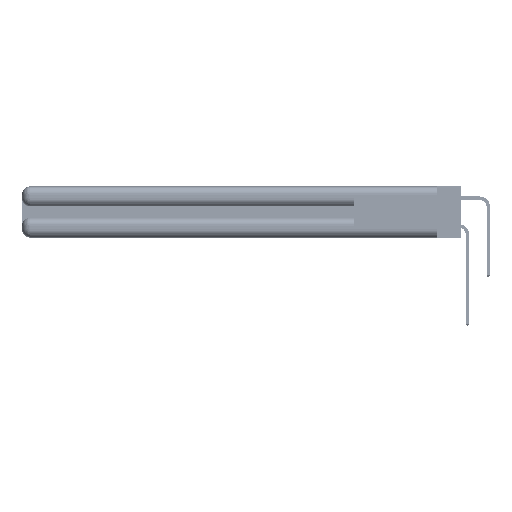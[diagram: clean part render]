
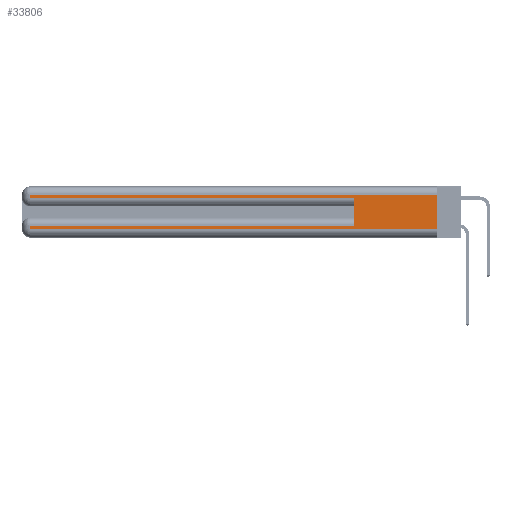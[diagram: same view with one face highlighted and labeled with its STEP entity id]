
A CAD part, left-side view. The second image highlights one B-rep face of the part: STEP entity #33806.
In plain terms, the highlighted planar face has unit normal (-1, 0, 0).
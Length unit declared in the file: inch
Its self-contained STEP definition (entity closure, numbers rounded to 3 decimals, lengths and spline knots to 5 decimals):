
#61 = CARTESIAN_POINT ( 'NONE',  ( 0., 0., 0.085 ) ) ;
#611 = LINE ( 'NONE', #39825, #20318 ) ;
#1524 = EDGE_CURVE ( 'NONE', #49992, #50321, #36615, .T. ) ;
#2165 = VECTOR ( 'NONE', #7806, 39.37008 ) ;
#2235 = VERTEX_POINT ( 'NONE', #43183 ) ;
#3613 = VERTEX_POINT ( 'NONE', #47721 ) ;
#4469 = EDGE_CURVE ( 'NONE', #2235, #3613, #46664, .T. ) ;
#4702 = VERTEX_POINT ( 'NONE', #43395 ) ;
#5149 = VECTOR ( 'NONE', #7594, 39.37008 ) ;
#6120 = EDGE_CURVE ( 'NONE', #3613, #20665, #23684, .T. ) ;
#7594 = DIRECTION ( 'NONE',  ( 0., 0., -1. ) ) ;
#7806 = DIRECTION ( 'NONE',  ( 0., 0., -1. ) ) ;
#8091 = FACE_OUTER_BOUND ( 'NONE', #41782, .T. ) ;
#8268 = DIRECTION ( 'NONE',  ( 0., 0., 1. ) ) ;
#9815 = ORIENTED_EDGE ( 'NONE', *, *, #10046, .T. ) ;
#9983 = DIRECTION ( 'NONE',  ( 0., 0., -1. ) ) ;
#10046 = EDGE_CURVE ( 'NONE', #4702, #2235, #33859, .T. ) ;
#13178 = VECTOR ( 'NONE', #44785, 39.37008 ) ;
#14245 = VECTOR ( 'NONE', #27651, 39.37008 ) ;
#15212 = VECTOR ( 'NONE', #9983, 39.37008 ) ;
#15981 = LINE ( 'NONE', #17790, #35748 ) ;
#17790 = CARTESIAN_POINT ( 'NONE',  ( 0., 0., 0.06 ) ) ;
#18642 = DIRECTION ( 'NONE',  ( 1., 0., 0. ) ) ;
#19459 = CARTESIAN_POINT ( 'NONE',  ( 0., 2.94, 0.06 ) ) ;
#20318 = VECTOR ( 'NONE', #8268, 39.37008 ) ;
#20665 = VERTEX_POINT ( 'NONE', #40956 ) ;
#23128 = LINE ( 'NONE', #43286, #2165 ) ;
#23350 = VECTOR ( 'NONE', #27715, 39.37008 ) ;
#23577 = ORIENTED_EDGE ( 'NONE', *, *, #43489, .T. ) ;
#23684 = LINE ( 'NONE', #25168, #13178 ) ;
#24715 = VERTEX_POINT ( 'NONE', #31631 ) ;
#25168 = CARTESIAN_POINT ( 'NONE',  ( 0., 0., 0.285 ) ) ;
#26271 = ORIENTED_EDGE ( 'NONE', *, *, #27307, .F. ) ;
#27306 = ORIENTED_EDGE ( 'NONE', *, *, #4469, .T. ) ;
#27307 = EDGE_CURVE ( 'NONE', #24715, #20665, #611, .T. ) ;
#27651 = DIRECTION ( 'NONE',  ( 0., 1., 0. ) ) ;
#27715 = DIRECTION ( 'NONE',  ( 0., 1., 0. ) ) ;
#29577 = ORIENTED_EDGE ( 'NONE', *, *, #39506, .T. ) ;
#31631 = CARTESIAN_POINT ( 'NONE',  ( 0., 0.6, 0.085 ) ) ;
#33377 = ORIENTED_EDGE ( 'NONE', *, *, #1524, .T. ) ;
#33462 = CARTESIAN_POINT ( 'NONE',  ( 0., 2.94, 0.085 ) ) ;
#33806 = ADVANCED_FACE ( 'NONE', ( #8091 ), #34363, .F. ) ;
#33859 = LINE ( 'NONE', #47305, #23350 ) ;
#34363 = PLANE ( 'NONE',  #47307 ) ;
#35031 = CARTESIAN_POINT ( 'NONE',  ( 0., 2.94, 0.37 ) ) ;
#35117 = CARTESIAN_POINT ( 'NONE',  ( 0., 0., 0.06 ) ) ;
#35748 = VECTOR ( 'NONE', #45357, 39.37008 ) ;
#36615 = LINE ( 'NONE', #35031, #5149 ) ;
#37460 = EDGE_CURVE ( 'NONE', #4702, #47340, #23128, .T. ) ;
#38318 = CARTESIAN_POINT ( 'NONE',  ( 0., 0., 0.37 ) ) ;
#39506 = EDGE_CURVE ( 'NONE', #24715, #49992, #45708, .T. ) ;
#39825 = CARTESIAN_POINT ( 'NONE',  ( 0., 0.6, 0.145 ) ) ;
#40956 = CARTESIAN_POINT ( 'NONE',  ( 0., 0.6, 0.285 ) ) ;
#41782 = EDGE_LOOP ( 'NONE', ( #46566, #9815, #27306, #47711, #26271, #29577, #33377, #23577 ) ) ;
#43183 = CARTESIAN_POINT ( 'NONE',  ( 0., 2.94, 0.31 ) ) ;
#43286 = CARTESIAN_POINT ( 'NONE',  ( 0., 0., 0.37 ) ) ;
#43395 = CARTESIAN_POINT ( 'NONE',  ( 0., 0., 0.31 ) ) ;
#43489 = EDGE_CURVE ( 'NONE', #50321, #47340, #15981, .T. ) ;
#44785 = DIRECTION ( 'NONE',  ( 0., -1., 0. ) ) ;
#45357 = DIRECTION ( 'NONE',  ( 0., -1., 0. ) ) ;
#45708 = LINE ( 'NONE', #61, #14245 ) ;
#46192 = DIRECTION ( 'NONE',  ( 0., 0., -1. ) ) ;
#46566 = ORIENTED_EDGE ( 'NONE', *, *, #37460, .F. ) ;
#46664 = LINE ( 'NONE', #49269, #15212 ) ;
#47305 = CARTESIAN_POINT ( 'NONE',  ( 0., 0., 0.31 ) ) ;
#47307 = AXIS2_PLACEMENT_3D ( 'NONE', #38318, #18642, #46192 ) ;
#47340 = VERTEX_POINT ( 'NONE', #35117 ) ;
#47711 = ORIENTED_EDGE ( 'NONE', *, *, #6120, .T. ) ;
#47721 = CARTESIAN_POINT ( 'NONE',  ( 0., 2.94, 0.285 ) ) ;
#49269 = CARTESIAN_POINT ( 'NONE',  ( 0., 2.94, 0.37 ) ) ;
#49992 = VERTEX_POINT ( 'NONE', #33462 ) ;
#50321 = VERTEX_POINT ( 'NONE', #19459 ) ;
